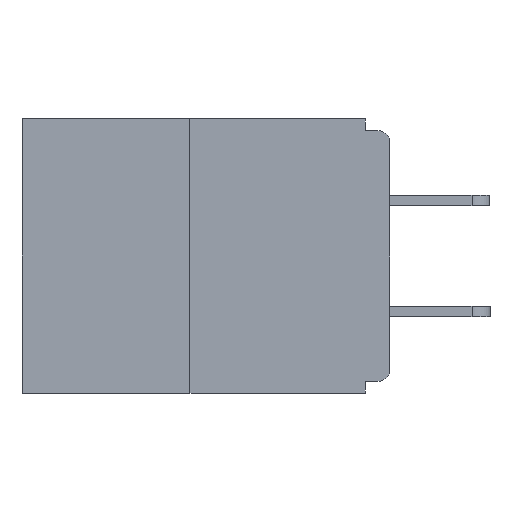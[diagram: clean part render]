
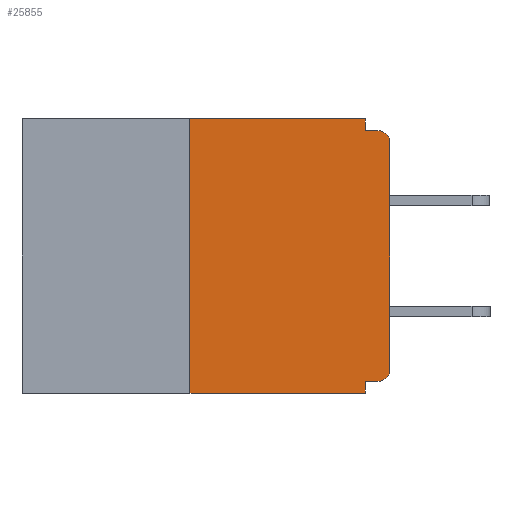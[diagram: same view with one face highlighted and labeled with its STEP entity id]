
A CAD part, left-side view. The second image highlights one B-rep face of the part: STEP entity #25855.
In plain terms, the highlighted planar face has unit normal (-1, 0, 0).
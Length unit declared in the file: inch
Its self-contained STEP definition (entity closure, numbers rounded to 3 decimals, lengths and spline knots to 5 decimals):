
#379 = CARTESIAN_POINT ( 'NONE',  ( 0., 0.015, -0.328 ) ) ;
#393 = LINE ( 'NONE', #1828, #26019 ) ;
#1608 = AXIS2_PLACEMENT_3D ( 'NONE', #16326, #16644, #6431 ) ;
#1665 = VECTOR ( 'NONE', #7318, 39.37008 ) ;
#1828 = CARTESIAN_POINT ( 'NONE',  ( 0., 0.46, 0. ) ) ;
#2029 = VECTOR ( 'NONE', #19783, 39.37008 ) ;
#2272 = LINE ( 'NONE', #4793, #13111 ) ;
#2799 = EDGE_CURVE ( 'NONE', #29546, #13050, #393, .T. ) ;
#2960 = VERTEX_POINT ( 'NONE', #379 ) ;
#3543 = ORIENTED_EDGE ( 'NONE', *, *, #9151, .T. ) ;
#3651 = CARTESIAN_POINT ( 'NONE',  ( 0., 0.031, -0.015 ) ) ;
#4144 = CIRCLE ( 'NONE', #18732, 0.015 ) ;
#4270 = LINE ( 'NONE', #8671, #22108 ) ;
#4793 = CARTESIAN_POINT ( 'NONE',  ( 0., 0.031, -0.343 ) ) ;
#4941 = CARTESIAN_POINT ( 'NONE',  ( 0., 0.015, -0.015 ) ) ;
#5122 = LINE ( 'NONE', #17621, #1665 ) ;
#6338 = ORIENTED_EDGE ( 'NONE', *, *, #6347, .T. ) ;
#6347 = EDGE_CURVE ( 'NONE', #29920, #9960, #5122, .T. ) ;
#6431 = DIRECTION ( 'NONE',  ( 0., 0., -1. ) ) ;
#6438 = ORIENTED_EDGE ( 'NONE', *, *, #7920, .F. ) ;
#6940 = AXIS2_PLACEMENT_3D ( 'NONE', #6973, #9483, #26858 ) ;
#6973 = CARTESIAN_POINT ( 'NONE',  ( 0., 0.015, -0.03 ) ) ;
#7318 = DIRECTION ( 'NONE',  ( 0., 0., 1. ) ) ;
#7455 = LINE ( 'NONE', #10044, #26479 ) ;
#7920 = EDGE_CURVE ( 'NONE', #22423, #29546, #11602, .T. ) ;
#8317 = EDGE_CURVE ( 'NONE', #24761, #13837, #2272, .T. ) ;
#8671 = CARTESIAN_POINT ( 'NONE',  ( 0., 0.46, -0.343 ) ) ;
#9151 = EDGE_CURVE ( 'NONE', #2960, #29920, #4144, .T. ) ;
#9211 = CARTESIAN_POINT ( 'NONE',  ( 0., 0.25, -0.343 ) ) ;
#9483 = DIRECTION ( 'NONE',  ( -1., 0., 0. ) ) ;
#9960 = VERTEX_POINT ( 'NONE', #18691 ) ;
#10044 = CARTESIAN_POINT ( 'NONE',  ( 0., 0., -0.015 ) ) ;
#10173 = LINE ( 'NONE', #31832, #2029 ) ;
#11602 = LINE ( 'NONE', #24820, #22446 ) ;
#11896 = CARTESIAN_POINT ( 'NONE',  ( 0., 0.031, 0. ) ) ;
#12167 = EDGE_CURVE ( 'NONE', #13050, #19139, #28283, .T. ) ;
#12523 = DIRECTION ( 'NONE',  ( 0., -1., 0. ) ) ;
#12849 = ORIENTED_EDGE ( 'NONE', *, *, #21692, .F. ) ;
#13050 = VERTEX_POINT ( 'NONE', #11896 ) ;
#13089 = CARTESIAN_POINT ( 'NONE',  ( 0., 0.25, 0. ) ) ;
#13111 = VECTOR ( 'NONE', #24428, 39.37008 ) ;
#13837 = VERTEX_POINT ( 'NONE', #31299 ) ;
#14050 = PLANE ( 'NONE',  #1608 ) ;
#14996 = ORIENTED_EDGE ( 'NONE', *, *, #12167, .F. ) ;
#16321 = CARTESIAN_POINT ( 'NONE',  ( 0., 0., -0.313 ) ) ;
#16326 = CARTESIAN_POINT ( 'NONE',  ( 0., 0.46, 0. ) ) ;
#16593 = VERTEX_POINT ( 'NONE', #4941 ) ;
#16644 = DIRECTION ( 'NONE',  ( 1., 0., 0. ) ) ;
#17621 = CARTESIAN_POINT ( 'NONE',  ( 0., 0., 0. ) ) ;
#17659 = ORIENTED_EDGE ( 'NONE', *, *, #21778, .F. ) ;
#18691 = CARTESIAN_POINT ( 'NONE',  ( 0., 0., -0.03 ) ) ;
#18732 = AXIS2_PLACEMENT_3D ( 'NONE', #21165, #18876, #21374 ) ;
#18876 = DIRECTION ( 'NONE',  ( -1., 0., 0. ) ) ;
#18987 = VECTOR ( 'NONE', #27261, 39.37008 ) ;
#19139 = VERTEX_POINT ( 'NONE', #3651 ) ;
#19783 = DIRECTION ( 'NONE',  ( 0., 1., 0. ) ) ;
#21165 = CARTESIAN_POINT ( 'NONE',  ( 0., 0.015, -0.313 ) ) ;
#21374 = DIRECTION ( 'NONE',  ( 0., 0., -1. ) ) ;
#21690 = ORIENTED_EDGE ( 'NONE', *, *, #2799, .F. ) ;
#21692 = EDGE_CURVE ( 'NONE', #2960, #24761, #10173, .T. ) ;
#21778 = EDGE_CURVE ( 'NONE', #19139, #16593, #7455, .T. ) ;
#22108 = VECTOR ( 'NONE', #28615, 39.37008 ) ;
#22423 = VERTEX_POINT ( 'NONE', #9211 ) ;
#22446 = VECTOR ( 'NONE', #24699, 39.37008 ) ;
#23105 = ORIENTED_EDGE ( 'NONE', *, *, #8317, .F. ) ;
#24428 = DIRECTION ( 'NONE',  ( 0., 0., -1. ) ) ;
#24699 = DIRECTION ( 'NONE',  ( 0., 0., 1. ) ) ;
#24761 = VERTEX_POINT ( 'NONE', #31798 ) ;
#24820 = CARTESIAN_POINT ( 'NONE',  ( 0., 0.25, 0. ) ) ;
#25855 = ADVANCED_FACE ( 'NONE', ( #26984 ), #14050, .F. ) ;
#26019 = VECTOR ( 'NONE', #31269, 39.37008 ) ;
#26188 = EDGE_LOOP ( 'NONE', ( #21690, #6438, #30503, #23105, #12849, #3543, #6338, #31250, #17659, #14996 ) ) ;
#26479 = VECTOR ( 'NONE', #12523, 39.37008 ) ;
#26858 = DIRECTION ( 'NONE',  ( 0., 0., -1. ) ) ;
#26984 = FACE_OUTER_BOUND ( 'NONE', #26188, .T. ) ;
#27261 = DIRECTION ( 'NONE',  ( 0., 0., -1. ) ) ;
#27745 = EDGE_CURVE ( 'NONE', #22423, #13837, #4270, .T. ) ;
#28283 = LINE ( 'NONE', #31990, #18987 ) ;
#28615 = DIRECTION ( 'NONE',  ( 0., -1., 0. ) ) ;
#29546 = VERTEX_POINT ( 'NONE', #13089 ) ;
#29920 = VERTEX_POINT ( 'NONE', #16321 ) ;
#30057 = EDGE_CURVE ( 'NONE', #9960, #16593, #31483, .T. ) ;
#30503 = ORIENTED_EDGE ( 'NONE', *, *, #27745, .T. ) ;
#31250 = ORIENTED_EDGE ( 'NONE', *, *, #30057, .T. ) ;
#31269 = DIRECTION ( 'NONE',  ( 0., -1., 0. ) ) ;
#31299 = CARTESIAN_POINT ( 'NONE',  ( 0., 0.031, -0.343 ) ) ;
#31483 = CIRCLE ( 'NONE', #6940, 0.015 ) ;
#31798 = CARTESIAN_POINT ( 'NONE',  ( 0., 0.031, -0.328 ) ) ;
#31832 = CARTESIAN_POINT ( 'NONE',  ( 0., 0., -0.328 ) ) ;
#31990 = CARTESIAN_POINT ( 'NONE',  ( 0., 0.031, 0. ) ) ;
